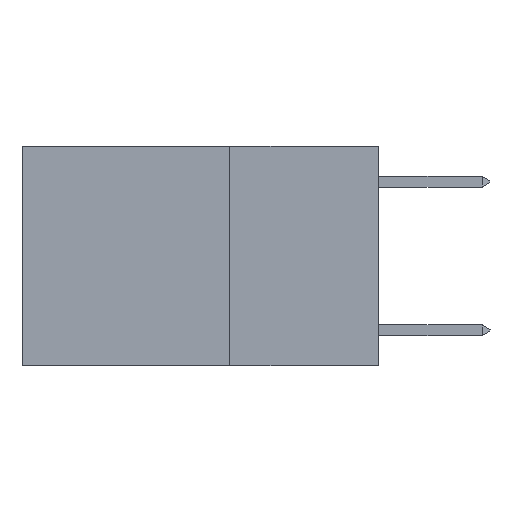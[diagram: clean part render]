
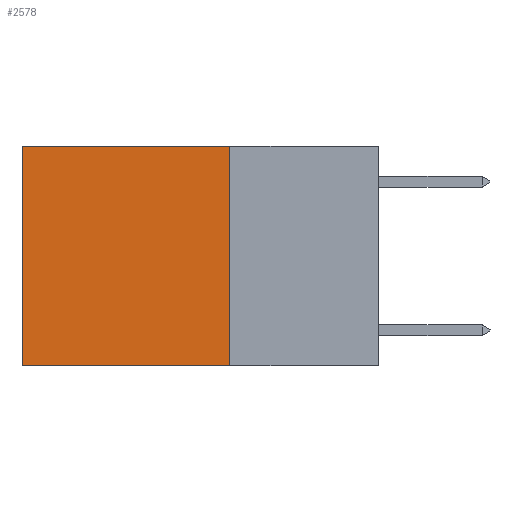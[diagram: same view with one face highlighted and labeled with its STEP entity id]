
A CAD part, left-side view. The second image highlights one B-rep face of the part: STEP entity #2578.
In plain terms, the highlighted planar face has unit normal (-1, 0, 0).
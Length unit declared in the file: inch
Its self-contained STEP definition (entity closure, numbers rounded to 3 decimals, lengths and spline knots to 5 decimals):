
#164 = DIRECTION ( 'NONE',  ( 0., 0., -1. ) ) ;
#299 = CARTESIAN_POINT ( 'NONE',  ( 0.2625, 0.6, 0. ) ) ;
#577 = AXIS2_PLACEMENT_3D ( 'NONE', #20906, #19978, #19854 ) ;
#1512 = VERTEX_POINT ( 'NONE', #10803 ) ;
#2535 = EDGE_CURVE ( 'NONE', #18252, #14036, #16648, .T. ) ;
#2578 = ADVANCED_FACE ( 'NONE', ( #17241 ), #20944, .F. ) ;
#4144 = ORIENTED_EDGE ( 'NONE', *, *, #2535, .T. ) ;
#6464 = DIRECTION ( 'NONE',  ( 0., 1., 0. ) ) ;
#6817 = ORIENTED_EDGE ( 'NONE', *, *, #20355, .T. ) ;
#9933 = DIRECTION ( 'NONE',  ( 0., 1., 0. ) ) ;
#10057 = CARTESIAN_POINT ( 'NONE',  ( 0.2625, 0.25, -0.37 ) ) ;
#10803 = CARTESIAN_POINT ( 'NONE',  ( 0.2625, 0.6, -0.37 ) ) ;
#11053 = EDGE_LOOP ( 'NONE', ( #6817, #14418, #12787, #4144 ) ) ;
#11819 = VECTOR ( 'NONE', #9933, 39.37008 ) ;
#11909 = VERTEX_POINT ( 'NONE', #18672 ) ;
#12127 = LINE ( 'NONE', #10057, #11819 ) ;
#12364 = CARTESIAN_POINT ( 'NONE',  ( 0.2625, 0.25, 0. ) ) ;
#12754 = EDGE_CURVE ( 'NONE', #11909, #1512, #12127, .T. ) ;
#12787 = ORIENTED_EDGE ( 'NONE', *, *, #15051, .F. ) ;
#13061 = CARTESIAN_POINT ( 'NONE',  ( 0.2625, 0.25, 0. ) ) ;
#14036 = VERTEX_POINT ( 'NONE', #14304 ) ;
#14164 = VECTOR ( 'NONE', #164, 39.37008 ) ;
#14304 = CARTESIAN_POINT ( 'NONE',  ( 0.2625, 0.6, 0. ) ) ;
#14418 = ORIENTED_EDGE ( 'NONE', *, *, #12754, .F. ) ;
#14428 = LINE ( 'NONE', #299, #14164 ) ;
#14890 = DIRECTION ( 'NONE',  ( 0., 0., -1. ) ) ;
#15051 = EDGE_CURVE ( 'NONE', #18252, #11909, #19561, .T. ) ;
#15392 = CARTESIAN_POINT ( 'NONE',  ( 0.2625, 0.25, 0. ) ) ;
#16648 = LINE ( 'NONE', #12364, #16930 ) ;
#16930 = VECTOR ( 'NONE', #6464, 39.37008 ) ;
#17241 = FACE_OUTER_BOUND ( 'NONE', #11053, .T. ) ;
#18252 = VERTEX_POINT ( 'NONE', #13061 ) ;
#18672 = CARTESIAN_POINT ( 'NONE',  ( 0.2625, 0.25, -0.37 ) ) ;
#19269 = VECTOR ( 'NONE', #14890, 39.37008 ) ;
#19561 = LINE ( 'NONE', #15392, #19269 ) ;
#19854 = DIRECTION ( 'NONE',  ( 0., 0., -1. ) ) ;
#19978 = DIRECTION ( 'NONE',  ( 1., 0., 0. ) ) ;
#20355 = EDGE_CURVE ( 'NONE', #14036, #1512, #14428, .T. ) ;
#20906 = CARTESIAN_POINT ( 'NONE',  ( 0.2625, 0.25, 0. ) ) ;
#20944 = PLANE ( 'NONE',  #577 ) ;
